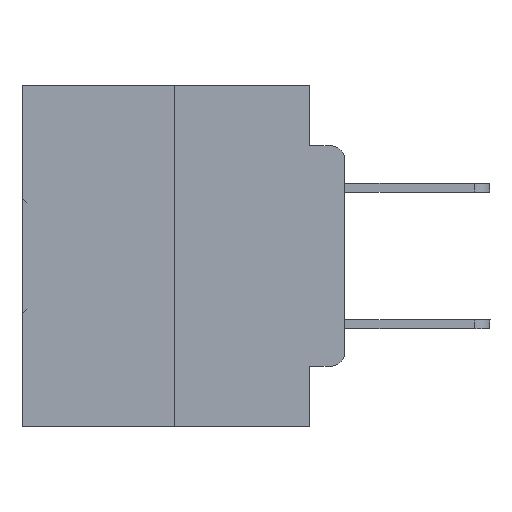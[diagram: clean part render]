
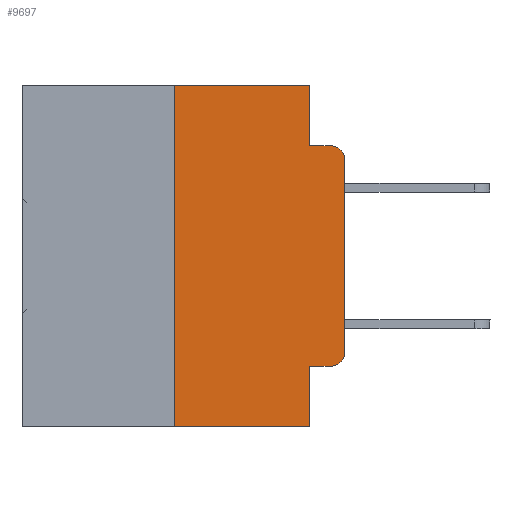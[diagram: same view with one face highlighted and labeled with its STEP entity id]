
A CAD part, left-side view. The second image highlights one B-rep face of the part: STEP entity #9697.
In plain terms, the highlighted planar face has unit normal (-1, 0, 0).
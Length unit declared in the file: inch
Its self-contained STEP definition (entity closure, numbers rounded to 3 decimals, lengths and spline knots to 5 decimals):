
#320 = CARTESIAN_POINT ( 'NONE',  ( 0., 0.051, -0.4115 ) ) ;
#1547 = CARTESIAN_POINT ( 'NONE',  ( 0., 0., 0. ) ) ;
#1587 = VECTOR ( 'NONE', #4840, 39.37008 ) ;
#2187 = EDGE_CURVE ( 'NONE', #24671, #24693, #4533, .T. ) ;
#3664 = EDGE_CURVE ( 'NONE', #27233, #12494, #20733, .T. ) ;
#4267 = ORIENTED_EDGE ( 'NONE', *, *, #13141, .F. ) ;
#4533 = CIRCLE ( 'NONE', #30519, 0.02 ) ;
#4840 = DIRECTION ( 'NONE',  ( 0., 0., -1. ) ) ;
#6689 = CARTESIAN_POINT ( 'NONE',  ( 0., 0.02, -0.4115 ) ) ;
#6733 = CARTESIAN_POINT ( 'NONE',  ( 0., 0.02, -0.1085 ) ) ;
#7078 = CARTESIAN_POINT ( 'NONE',  ( 0., 0.25, 0. ) ) ;
#7291 = CARTESIAN_POINT ( 'NONE',  ( 0., 0.051, -0.0885 ) ) ;
#7452 = VECTOR ( 'NONE', #25478, 39.37008 ) ;
#8585 = CARTESIAN_POINT ( 'NONE',  ( 0., 0.473, 0. ) ) ;
#9657 = VERTEX_POINT ( 'NONE', #11811 ) ;
#9697 = ADVANCED_FACE ( 'NONE', ( #28118 ), #33842, .F. ) ;
#9890 = DIRECTION ( 'NONE',  ( 0., -1., 0. ) ) ;
#10264 = DIRECTION ( 'NONE',  ( 0., 0., -1. ) ) ;
#10577 = ORIENTED_EDGE ( 'NONE', *, *, #3664, .F. ) ;
#10897 = DIRECTION ( 'NONE',  ( 0., -1., 0. ) ) ;
#11811 = CARTESIAN_POINT ( 'NONE',  ( 0., 0.051, -0.5 ) ) ;
#12054 = CARTESIAN_POINT ( 'NONE',  ( 0., 0.02, -0.0885 ) ) ;
#12283 = CARTESIAN_POINT ( 'NONE',  ( 0., 0.051, 0. ) ) ;
#12437 = ORIENTED_EDGE ( 'NONE', *, *, #30735, .T. ) ;
#12494 = VERTEX_POINT ( 'NONE', #31794 ) ;
#12602 = CARTESIAN_POINT ( 'NONE',  ( 0., 0., -0.3915 ) ) ;
#12696 = EDGE_CURVE ( 'NONE', #12494, #23216, #22895, .T. ) ;
#13141 = EDGE_CURVE ( 'NONE', #18426, #17389, #31358, .T. ) ;
#13194 = CARTESIAN_POINT ( 'NONE',  ( 0., 0., -0.1085 ) ) ;
#13309 = ORIENTED_EDGE ( 'NONE', *, *, #31389, .F. ) ;
#13407 = EDGE_CURVE ( 'NONE', #28476, #24671, #28761, .T. ) ;
#13661 = AXIS2_PLACEMENT_3D ( 'NONE', #23260, #26041, #10264 ) ;
#15067 = LINE ( 'NONE', #12283, #1587 ) ;
#15470 = VECTOR ( 'NONE', #9890, 39.37008 ) ;
#15552 = ORIENTED_EDGE ( 'NONE', *, *, #19284, .T. ) ;
#15825 = ORIENTED_EDGE ( 'NONE', *, *, #13407, .T. ) ;
#16285 = ORIENTED_EDGE ( 'NONE', *, *, #25423, .F. ) ;
#16395 = DIRECTION ( 'NONE',  ( 0., -1., 0. ) ) ;
#16557 = AXIS2_PLACEMENT_3D ( 'NONE', #6733, #21543, #29992 ) ;
#17389 = VERTEX_POINT ( 'NONE', #33425 ) ;
#17409 = CARTESIAN_POINT ( 'NONE',  ( 0., 0.473, -0.5 ) ) ;
#17494 = DIRECTION ( 'NONE',  ( 0., 0., 1. ) ) ;
#17750 = DIRECTION ( 'NONE',  ( 0., -1., 0. ) ) ;
#18426 = VERTEX_POINT ( 'NONE', #30762 ) ;
#18549 = CARTESIAN_POINT ( 'NONE',  ( 0., 0.02, -0.3915 ) ) ;
#19010 = LINE ( 'NONE', #8585, #23604 ) ;
#19284 = EDGE_CURVE ( 'NONE', #24693, #29555, #27899, .T. ) ;
#20257 = CARTESIAN_POINT ( 'NONE',  ( 0., 0.051, -0.4115 ) ) ;
#20475 = VECTOR ( 'NONE', #17494, 39.37008 ) ;
#20733 = LINE ( 'NONE', #29060, #30622 ) ;
#20999 = CIRCLE ( 'NONE', #16557, 0.02 ) ;
#21543 = DIRECTION ( 'NONE',  ( -1., 0., 0. ) ) ;
#21983 = EDGE_LOOP ( 'NONE', ( #15552, #31911, #25715, #10577, #13309, #4267, #12437, #16285, #15825, #25900 ) ) ;
#22662 = CARTESIAN_POINT ( 'NONE',  ( 0., 0.051, 0. ) ) ;
#22895 = LINE ( 'NONE', #7291, #15470 ) ;
#23216 = VERTEX_POINT ( 'NONE', #12054 ) ;
#23260 = CARTESIAN_POINT ( 'NONE',  ( 0., 0.473, 0. ) ) ;
#23604 = VECTOR ( 'NONE', #16395, 39.37008 ) ;
#24083 = DIRECTION ( 'NONE',  ( -1., 0., 0. ) ) ;
#24671 = VERTEX_POINT ( 'NONE', #6689 ) ;
#24693 = VERTEX_POINT ( 'NONE', #12602 ) ;
#25365 = EDGE_CURVE ( 'NONE', #29555, #23216, #20999, .T. ) ;
#25423 = EDGE_CURVE ( 'NONE', #28476, #9657, #15067, .T. ) ;
#25478 = DIRECTION ( 'NONE',  ( 0., 0., 1. ) ) ;
#25715 = ORIENTED_EDGE ( 'NONE', *, *, #12696, .F. ) ;
#25900 = ORIENTED_EDGE ( 'NONE', *, *, #2187, .T. ) ;
#26041 = DIRECTION ( 'NONE',  ( 1., 0., 0. ) ) ;
#27233 = VERTEX_POINT ( 'NONE', #22662 ) ;
#27899 = LINE ( 'NONE', #1547, #7452 ) ;
#28118 = FACE_OUTER_BOUND ( 'NONE', #21983, .T. ) ;
#28476 = VERTEX_POINT ( 'NONE', #20257 ) ;
#28761 = LINE ( 'NONE', #320, #29906 ) ;
#29060 = CARTESIAN_POINT ( 'NONE',  ( 0., 0.051, 0. ) ) ;
#29555 = VERTEX_POINT ( 'NONE', #13194 ) ;
#29906 = VECTOR ( 'NONE', #10897, 39.37008 ) ;
#29992 = DIRECTION ( 'NONE',  ( 0., 0., -1. ) ) ;
#30254 = VECTOR ( 'NONE', #17750, 39.37008 ) ;
#30519 = AXIS2_PLACEMENT_3D ( 'NONE', #18549, #24083, #31894 ) ;
#30622 = VECTOR ( 'NONE', #31295, 39.37008 ) ;
#30735 = EDGE_CURVE ( 'NONE', #18426, #9657, #33171, .T. ) ;
#30762 = CARTESIAN_POINT ( 'NONE',  ( 0., 0.25, -0.5 ) ) ;
#31295 = DIRECTION ( 'NONE',  ( 0., 0., -1. ) ) ;
#31358 = LINE ( 'NONE', #7078, #20475 ) ;
#31389 = EDGE_CURVE ( 'NONE', #17389, #27233, #19010, .T. ) ;
#31794 = CARTESIAN_POINT ( 'NONE',  ( 0., 0.051, -0.0885 ) ) ;
#31894 = DIRECTION ( 'NONE',  ( 0., 0., -1. ) ) ;
#31911 = ORIENTED_EDGE ( 'NONE', *, *, #25365, .T. ) ;
#33171 = LINE ( 'NONE', #17409, #30254 ) ;
#33425 = CARTESIAN_POINT ( 'NONE',  ( 0., 0.25, 0. ) ) ;
#33842 = PLANE ( 'NONE',  #13661 ) ;
